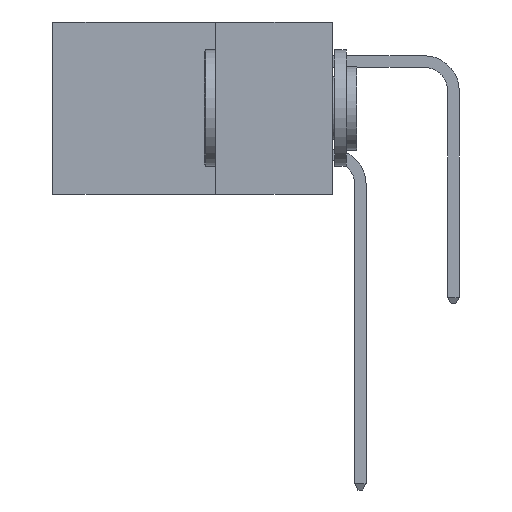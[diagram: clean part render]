
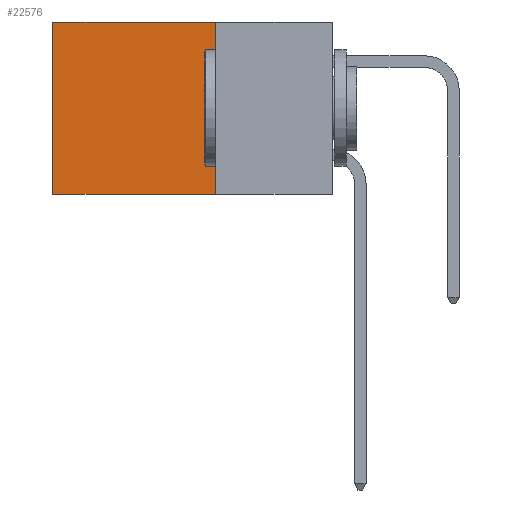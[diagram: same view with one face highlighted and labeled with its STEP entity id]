
A CAD part, left-side view. The second image highlights one B-rep face of the part: STEP entity #22576.
In plain terms, the highlighted planar face has unit normal (-1, 0, 0).
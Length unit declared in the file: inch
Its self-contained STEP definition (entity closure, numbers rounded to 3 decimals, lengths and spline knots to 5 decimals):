
#535 = DIRECTION ( 'NONE',  ( 0., 1., 0. ) ) ;
#1610 = AXIS2_PLACEMENT_3D ( 'NONE', #13024, #15150, #2339 ) ;
#2339 = DIRECTION ( 'NONE',  ( 0., 0., -1. ) ) ;
#2429 = DIRECTION ( 'NONE',  ( 0., 1., 0. ) ) ;
#2545 = CARTESIAN_POINT ( 'NONE',  ( 0.2615, 0.25, 0. ) ) ;
#2662 = LINE ( 'NONE', #9656, #13387 ) ;
#3289 = ORIENTED_EDGE ( 'NONE', *, *, #4925, .F. ) ;
#3957 = FACE_OUTER_BOUND ( 'NONE', #24079, .T. ) ;
#4067 = CARTESIAN_POINT ( 'NONE',  ( 0.2615, 0.25, -0.37 ) ) ;
#4925 = EDGE_CURVE ( 'NONE', #8127, #15874, #21672, .T. ) ;
#5404 = DIRECTION ( 'NONE',  ( 0., 0., -1. ) ) ;
#6528 = CARTESIAN_POINT ( 'NONE',  ( 0.2615, 0.25, -0.37 ) ) ;
#7467 = ORIENTED_EDGE ( 'NONE', *, *, #22195, .T. ) ;
#7582 = CARTESIAN_POINT ( 'NONE',  ( 0.2615, 0.25, -0.37 ) ) ;
#7757 = EDGE_CURVE ( 'NONE', #11990, #8127, #23777, .T. ) ;
#8127 = VERTEX_POINT ( 'NONE', #6528 ) ;
#9473 = ORIENTED_EDGE ( 'NONE', *, *, #7757, .F. ) ;
#9656 = CARTESIAN_POINT ( 'NONE',  ( 0.2615, 0.6, -0.37 ) ) ;
#9754 = DIRECTION ( 'NONE',  ( 0., 0., -1. ) ) ;
#10370 = CARTESIAN_POINT ( 'NONE',  ( 0.2615, 0.6, 0. ) ) ;
#10389 = VECTOR ( 'NONE', #2429, 39.37008 ) ;
#10526 = CARTESIAN_POINT ( 'NONE',  ( 0.2615, 0.6, -0.37 ) ) ;
#10782 = VECTOR ( 'NONE', #535, 39.37008 ) ;
#11449 = LINE ( 'NONE', #21889, #10782 ) ;
#11562 = ORIENTED_EDGE ( 'NONE', *, *, #23923, .T. ) ;
#11990 = VERTEX_POINT ( 'NONE', #2545 ) ;
#12565 = VECTOR ( 'NONE', #9754, 39.37008 ) ;
#13024 = CARTESIAN_POINT ( 'NONE',  ( 0.2615, 0.25, -0.37 ) ) ;
#13387 = VECTOR ( 'NONE', #5404, 39.37008 ) ;
#15150 = DIRECTION ( 'NONE',  ( 1., 0., 0. ) ) ;
#15874 = VERTEX_POINT ( 'NONE', #10526 ) ;
#21672 = LINE ( 'NONE', #4067, #10389 ) ;
#21889 = CARTESIAN_POINT ( 'NONE',  ( 0.2615, 0.25, 0. ) ) ;
#22195 = EDGE_CURVE ( 'NONE', #24265, #15874, #2662, .T. ) ;
#22576 = ADVANCED_FACE ( 'NONE', ( #3957 ), #25588, .F. ) ;
#23777 = LINE ( 'NONE', #7582, #12565 ) ;
#23923 = EDGE_CURVE ( 'NONE', #11990, #24265, #11449, .T. ) ;
#24079 = EDGE_LOOP ( 'NONE', ( #7467, #3289, #9473, #11562 ) ) ;
#24265 = VERTEX_POINT ( 'NONE', #10370 ) ;
#25588 = PLANE ( 'NONE',  #1610 ) ;
